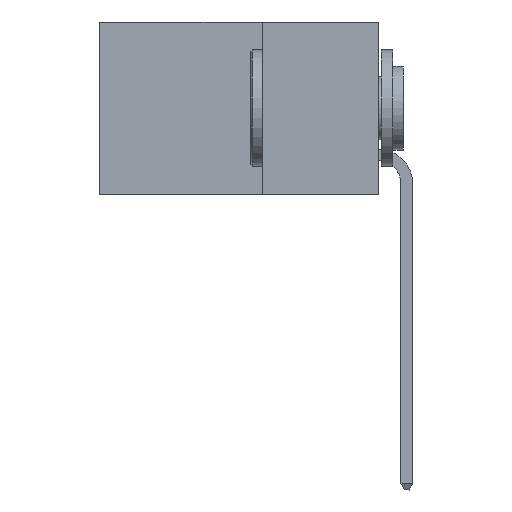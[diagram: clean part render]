
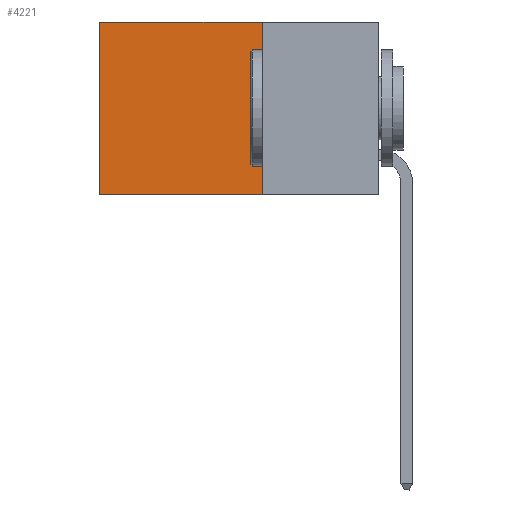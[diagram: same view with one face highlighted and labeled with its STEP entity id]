
A CAD part, left-side view. The second image highlights one B-rep face of the part: STEP entity #4221.
In plain terms, the highlighted planar face has unit normal (-1, 0, 0).
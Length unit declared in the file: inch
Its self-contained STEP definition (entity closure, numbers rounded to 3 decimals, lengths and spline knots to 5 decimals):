
#1170 = VERTEX_POINT ( 'NONE', #5055 ) ;
#1437 = CARTESIAN_POINT ( 'NONE',  ( 0.298, 0.6, 0. ) ) ;
#1476 = CARTESIAN_POINT ( 'NONE',  ( 0.298, 0.6, -0.37 ) ) ;
#1522 = EDGE_CURVE ( 'NONE', #1170, #1550, #5549, .T. ) ;
#1550 = VERTEX_POINT ( 'NONE', #1476 ) ;
#2099 = ORIENTED_EDGE ( 'NONE', *, *, #4123, .T. ) ;
#2201 = FACE_OUTER_BOUND ( 'NONE', #4012, .T. ) ;
#2283 = VECTOR ( 'NONE', #6817, 39.37008 ) ;
#2885 = DIRECTION ( 'NONE',  ( 1., 0., 0. ) ) ;
#3134 = VECTOR ( 'NONE', #3422, 39.37008 ) ;
#3188 = VERTEX_POINT ( 'NONE', #6929 ) ;
#3242 = CARTESIAN_POINT ( 'NONE',  ( 0.298, 0.25, 0. ) ) ;
#3322 = DIRECTION ( 'NONE',  ( 0., 0., -1. ) ) ;
#3354 = DIRECTION ( 'NONE',  ( 0., 1., 0. ) ) ;
#3422 = DIRECTION ( 'NONE',  ( 0., 1., 0. ) ) ;
#4012 = EDGE_LOOP ( 'NONE', ( #9595, #8534, #5213, #2099 ) ) ;
#4123 = EDGE_CURVE ( 'NONE', #3188, #8803, #5092, .T. ) ;
#4221 = ADVANCED_FACE ( 'NONE', ( #2201 ), #6086, .F. ) ;
#5012 = AXIS2_PLACEMENT_3D ( 'NONE', #7209, #2885, #3322 ) ;
#5055 = CARTESIAN_POINT ( 'NONE',  ( 0.298, 0.25, -0.37 ) ) ;
#5092 = LINE ( 'NONE', #3242, #8619 ) ;
#5213 = ORIENTED_EDGE ( 'NONE', *, *, #8982, .F. ) ;
#5549 = LINE ( 'NONE', #7293, #3134 ) ;
#5743 = VECTOR ( 'NONE', #9822, 39.37008 ) ;
#6086 = PLANE ( 'NONE',  #5012 ) ;
#6231 = LINE ( 'NONE', #7042, #2283 ) ;
#6817 = DIRECTION ( 'NONE',  ( 0., 0., -1. ) ) ;
#6833 = EDGE_CURVE ( 'NONE', #8803, #1550, #6231, .T. ) ;
#6929 = CARTESIAN_POINT ( 'NONE',  ( 0.298, 0.25, 0. ) ) ;
#7042 = CARTESIAN_POINT ( 'NONE',  ( 0.298, 0.6, 0. ) ) ;
#7209 = CARTESIAN_POINT ( 'NONE',  ( 0.298, 0.25, 0. ) ) ;
#7293 = CARTESIAN_POINT ( 'NONE',  ( 0.298, 0.25, -0.37 ) ) ;
#7513 = LINE ( 'NONE', #8435, #5743 ) ;
#8435 = CARTESIAN_POINT ( 'NONE',  ( 0.298, 0.25, 0. ) ) ;
#8534 = ORIENTED_EDGE ( 'NONE', *, *, #1522, .F. ) ;
#8619 = VECTOR ( 'NONE', #3354, 39.37008 ) ;
#8803 = VERTEX_POINT ( 'NONE', #1437 ) ;
#8982 = EDGE_CURVE ( 'NONE', #3188, #1170, #7513, .T. ) ;
#9595 = ORIENTED_EDGE ( 'NONE', *, *, #6833, .T. ) ;
#9822 = DIRECTION ( 'NONE',  ( 0., 0., -1. ) ) ;
